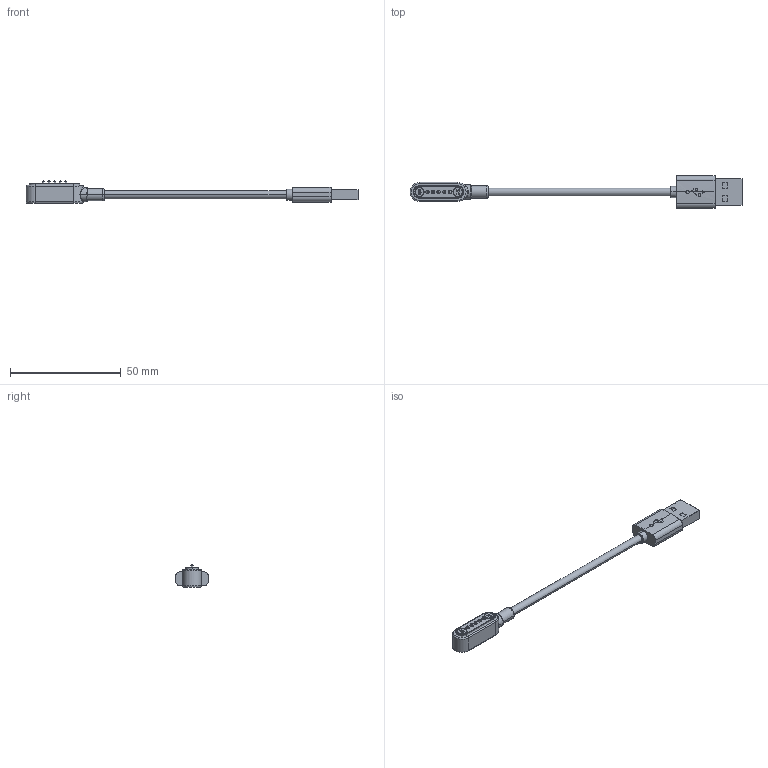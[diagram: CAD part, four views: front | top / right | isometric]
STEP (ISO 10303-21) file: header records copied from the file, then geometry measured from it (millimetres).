
FILE_DESCRIPTION (( 'STEP AP214' ), '1' );
FILE_NAME ('687D0522A510200.STEP', '2023-04-13T14:37:12', ( '' ), ( '' ), 'SwSTEP 2.0', 'SolidWorks 2020', '' );
FILE_SCHEMA (( 'AUTOMOTIVE_DESIGN' ));
Length unit declared in the file: millimetre
Products named in the file (1): 687D0522A510200
Bounding box: 150.06 x 14.8 x 10 mm (x, y, z)
Surface area: 5380.1 mm2 (no closed solid volume)
Topology: 0 solids, 3 shells, 419 faces, 1034 edges, 670 vertices
Faces by surface type: plane 175, cylinder 166, torus 46, bspline 32
Entity records: 19982 total; most frequent: CARTESIAN_POINT 5730, ORIENTED_EDGE 2068, DIRECTION 1852, EDGE_CURVE 1034, AXIS2_PLACEMENT_3D 724, VERTEX_POINT 670, EDGE_LOOP 500, UNCERTAINTY_MEASURE_WITH_UNIT 422
